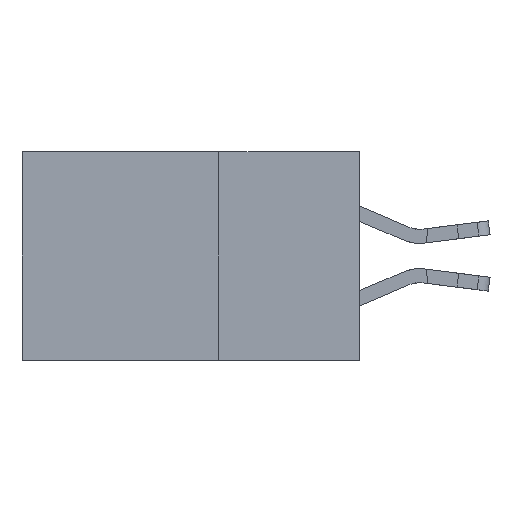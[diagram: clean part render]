
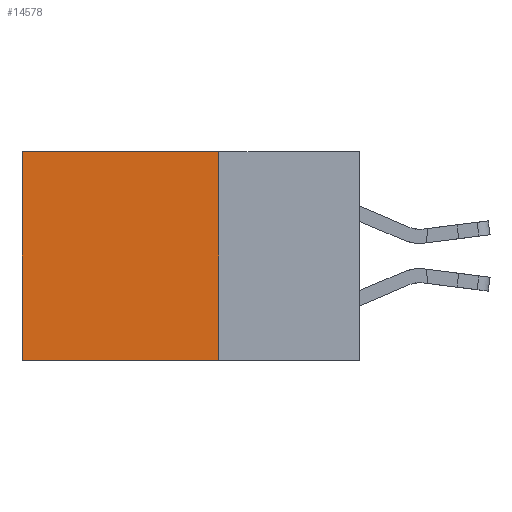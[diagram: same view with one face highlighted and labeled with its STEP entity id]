
A CAD part, left-side view. The second image highlights one B-rep face of the part: STEP entity #14578.
In plain terms, the highlighted planar face has unit normal (-1, 0, 0).
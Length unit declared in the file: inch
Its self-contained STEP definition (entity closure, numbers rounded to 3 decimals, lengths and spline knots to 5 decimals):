
#231 = VECTOR ( 'NONE', #10150, 39.37008 ) ;
#321 = CARTESIAN_POINT ( 'NONE',  ( 0.2875, 0.25, 0. ) ) ;
#423 = DIRECTION ( 'NONE',  ( 0., 1., 0. ) ) ;
#689 = VERTEX_POINT ( 'NONE', #5048 ) ;
#787 = EDGE_CURVE ( 'NONE', #8722, #4586, #8593, .T. ) ;
#923 = CARTESIAN_POINT ( 'NONE',  ( 0.2875, 0.25, -0.37 ) ) ;
#1032 = FACE_OUTER_BOUND ( 'NONE', #1113, .T. ) ;
#1113 = EDGE_LOOP ( 'NONE', ( #10343, #2335, #5595, #4682 ) ) ;
#2335 = ORIENTED_EDGE ( 'NONE', *, *, #9461, .F. ) ;
#2700 = DIRECTION ( 'NONE',  ( 1., 0., 0. ) ) ;
#3170 = CARTESIAN_POINT ( 'NONE',  ( 0.2875, 0.6, 0. ) ) ;
#4134 = EDGE_CURVE ( 'NONE', #689, #8722, #5665, .T. ) ;
#4586 = VERTEX_POINT ( 'NONE', #11141 ) ;
#4682 = ORIENTED_EDGE ( 'NONE', *, *, #4134, .T. ) ;
#5030 = LINE ( 'NONE', #923, #14558 ) ;
#5048 = CARTESIAN_POINT ( 'NONE',  ( 0.2875, 0.25, 0. ) ) ;
#5384 = LINE ( 'NONE', #6135, #12602 ) ;
#5595 = ORIENTED_EDGE ( 'NONE', *, *, #10271, .F. ) ;
#5665 = LINE ( 'NONE', #321, #6621 ) ;
#6135 = CARTESIAN_POINT ( 'NONE',  ( 0.2875, 0.25, 0. ) ) ;
#6621 = VECTOR ( 'NONE', #423, 39.37008 ) ;
#6789 = AXIS2_PLACEMENT_3D ( 'NONE', #9966, #2700, #14922 ) ;
#8358 = DIRECTION ( 'NONE',  ( 0., 1., 0. ) ) ;
#8593 = LINE ( 'NONE', #11113, #231 ) ;
#8722 = VERTEX_POINT ( 'NONE', #3170 ) ;
#9461 = EDGE_CURVE ( 'NONE', #13707, #4586, #5030, .T. ) ;
#9966 = CARTESIAN_POINT ( 'NONE',  ( 0.2875, 0.25, 0. ) ) ;
#10150 = DIRECTION ( 'NONE',  ( 0., 0., -1. ) ) ;
#10271 = EDGE_CURVE ( 'NONE', #689, #13707, #5384, .T. ) ;
#10343 = ORIENTED_EDGE ( 'NONE', *, *, #787, .T. ) ;
#10851 = CARTESIAN_POINT ( 'NONE',  ( 0.2875, 0.25, -0.37 ) ) ;
#11113 = CARTESIAN_POINT ( 'NONE',  ( 0.2875, 0.6, 0. ) ) ;
#11141 = CARTESIAN_POINT ( 'NONE',  ( 0.2875, 0.6, -0.37 ) ) ;
#12602 = VECTOR ( 'NONE', #13370, 39.37008 ) ;
#13370 = DIRECTION ( 'NONE',  ( 0., 0., -1. ) ) ;
#13707 = VERTEX_POINT ( 'NONE', #10851 ) ;
#13808 = PLANE ( 'NONE',  #6789 ) ;
#14558 = VECTOR ( 'NONE', #8358, 39.37008 ) ;
#14578 = ADVANCED_FACE ( 'NONE', ( #1032 ), #13808, .F. ) ;
#14922 = DIRECTION ( 'NONE',  ( 0., 0., -1. ) ) ;
